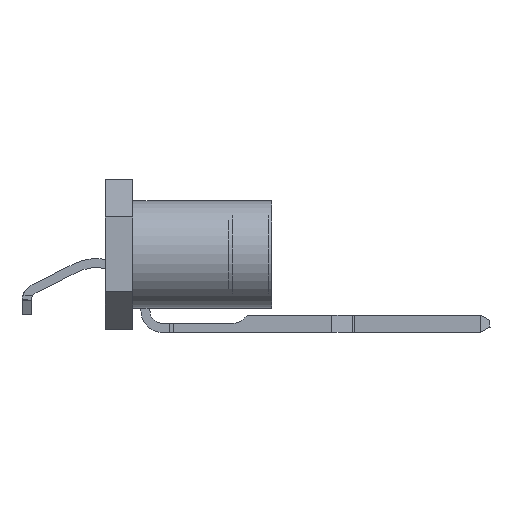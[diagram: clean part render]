
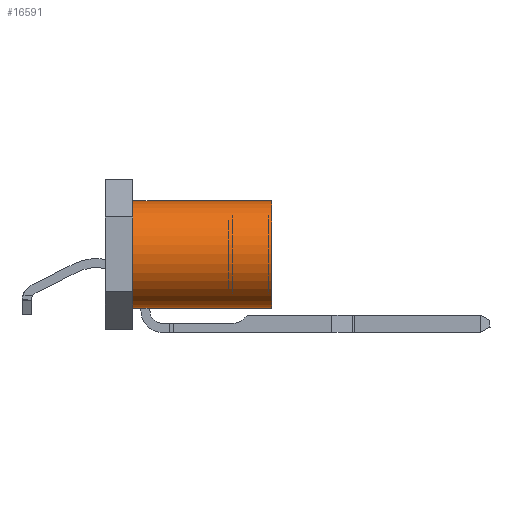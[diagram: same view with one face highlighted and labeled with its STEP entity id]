
A CAD part, left-side view. The second image highlights one B-rep face of the part: STEP entity #16591.
In plain terms, the highlighted cylindrical face has radius 1.968 mm (diameter 3.937 mm), a partial arc.
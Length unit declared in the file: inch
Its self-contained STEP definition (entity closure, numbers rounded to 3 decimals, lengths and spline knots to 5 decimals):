
#171 = AXIS2_PLACEMENT_3D ( 'NONE', #26887, #7565, #30080 ) ;
#985 = DIRECTION ( 'NONE',  ( 0., 0., -1. ) ) ;
#1957 = EDGE_CURVE ( 'NONE', #23837, #16083, #24831, .T. ) ;
#6181 = ORIENTED_EDGE ( 'NONE', *, *, #41327, .F. ) ;
#6406 = VECTOR ( 'NONE', #13625, 39.37008 ) ;
#7178 = DIRECTION ( 'NONE',  ( 0., 1., 0. ) ) ;
#7551 = VERTEX_POINT ( 'NONE', #14053 ) ;
#7565 = DIRECTION ( 'NONE',  ( 0., 1., 0. ) ) ;
#9016 = CARTESIAN_POINT ( 'NONE',  ( 0., 0.24, 0.0775 ) ) ;
#10424 = CARTESIAN_POINT ( 'NONE',  ( 0., 0.24, -0.0775 ) ) ;
#12186 = CARTESIAN_POINT ( 'NONE',  ( 0., 0.04, -0.0775 ) ) ;
#12856 = VECTOR ( 'NONE', #28290, 39.37008 ) ;
#13625 = DIRECTION ( 'NONE',  ( 0., -1., 0. ) ) ;
#14053 = CARTESIAN_POINT ( 'NONE',  ( 0., 0.24, 0.0775 ) ) ;
#14493 = VERTEX_POINT ( 'NONE', #16003 ) ;
#16003 = CARTESIAN_POINT ( 'NONE',  ( 0., 0.24, -0.0775 ) ) ;
#16083 = VERTEX_POINT ( 'NONE', #36552 ) ;
#16397 = FACE_OUTER_BOUND ( 'NONE', #28152, .T. ) ;
#16591 = ADVANCED_FACE ( 'NONE', ( #16397 ), #40977, .T. ) ;
#16900 = EDGE_CURVE ( 'NONE', #7551, #16083, #37458, .T. ) ;
#20324 = CARTESIAN_POINT ( 'NONE',  ( 0., 0.24, 0. ) ) ;
#22546 = ORIENTED_EDGE ( 'NONE', *, *, #41343, .T. ) ;
#23837 = VERTEX_POINT ( 'NONE', #12186 ) ;
#24831 = CIRCLE ( 'NONE', #171, 0.0775 ) ;
#26492 = CARTESIAN_POINT ( 'NONE',  ( 0., 0.24, 0. ) ) ;
#26887 = CARTESIAN_POINT ( 'NONE',  ( 0., 0.04, 0. ) ) ;
#28152 = EDGE_LOOP ( 'NONE', ( #37472, #6181, #22546, #35547 ) ) ;
#28290 = DIRECTION ( 'NONE',  ( 0., -1., 0. ) ) ;
#29683 = DIRECTION ( 'NONE',  ( 0., 0., 1. ) ) ;
#30080 = DIRECTION ( 'NONE',  ( 0., 0., 1. ) ) ;
#32072 = LINE ( 'NONE', #10424, #6406 ) ;
#35547 = ORIENTED_EDGE ( 'NONE', *, *, #1957, .T. ) ;
#36261 = DIRECTION ( 'NONE',  ( 0., -1., 0. ) ) ;
#36552 = CARTESIAN_POINT ( 'NONE',  ( 0., 0.04, 0.0775 ) ) ;
#37458 = LINE ( 'NONE', #9016, #12856 ) ;
#37472 = ORIENTED_EDGE ( 'NONE', *, *, #16900, .F. ) ;
#37806 = AXIS2_PLACEMENT_3D ( 'NONE', #20324, #36261, #985 ) ;
#40566 = CIRCLE ( 'NONE', #41587, 0.0775 ) ;
#40977 = CYLINDRICAL_SURFACE ( 'NONE', #37806, 0.0775 ) ;
#41327 = EDGE_CURVE ( 'NONE', #14493, #7551, #40566, .T. ) ;
#41343 = EDGE_CURVE ( 'NONE', #14493, #23837, #32072, .T. ) ;
#41587 = AXIS2_PLACEMENT_3D ( 'NONE', #26492, #7178, #29683 ) ;
